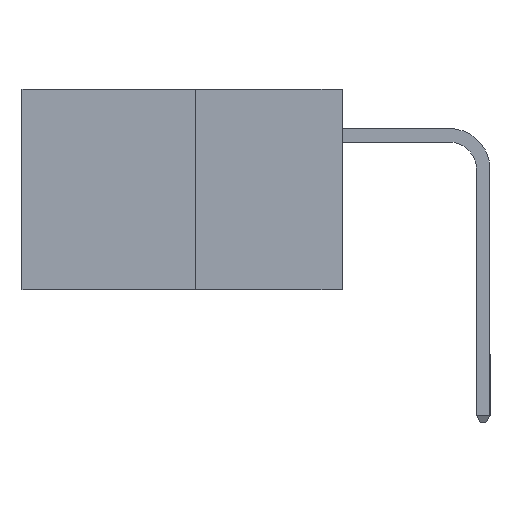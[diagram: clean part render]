
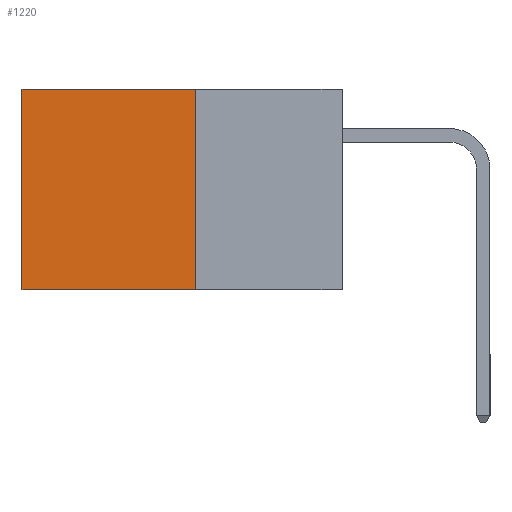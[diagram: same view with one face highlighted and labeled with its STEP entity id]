
A CAD part, left-side view. The second image highlights one B-rep face of the part: STEP entity #1220.
In plain terms, the highlighted planar face has unit normal (-1, 0, 0).
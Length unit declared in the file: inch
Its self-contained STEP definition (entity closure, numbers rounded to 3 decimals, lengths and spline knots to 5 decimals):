
#165 = LINE ( 'NONE', #10341, #7645 ) ;
#206 = CARTESIAN_POINT ( 'NONE',  ( 0.277, 0.27, -0.37 ) ) ;
#875 = EDGE_CURVE ( 'NONE', #8122, #924, #165, .T. ) ;
#924 = VERTEX_POINT ( 'NONE', #4427 ) ;
#1058 = ORIENTED_EDGE ( 'NONE', *, *, #8032, .T. ) ;
#1220 = ADVANCED_FACE ( 'NONE', ( #4016 ), #4090, .F. ) ;
#1400 = DIRECTION ( 'NONE',  ( 0., 0., -1. ) ) ;
#1431 = DIRECTION ( 'NONE',  ( 1., 0., 0. ) ) ;
#1976 = ORIENTED_EDGE ( 'NONE', *, *, #875, .F. ) ;
#2445 = LINE ( 'NONE', #11500, #9314 ) ;
#2619 = VECTOR ( 'NONE', #3828, 39.37008 ) ;
#2685 = AXIS2_PLACEMENT_3D ( 'NONE', #206, #1431, #1400 ) ;
#3040 = LINE ( 'NONE', #6504, #5522 ) ;
#3828 = DIRECTION ( 'NONE',  ( 0., 1., 0. ) ) ;
#4016 = FACE_OUTER_BOUND ( 'NONE', #5751, .T. ) ;
#4090 = PLANE ( 'NONE',  #2685 ) ;
#4427 = CARTESIAN_POINT ( 'NONE',  ( 0.277, 0.27, -0.37 ) ) ;
#4840 = CARTESIAN_POINT ( 'NONE',  ( 0.277, 0.27, 0. ) ) ;
#5522 = VECTOR ( 'NONE', #7401, 39.37008 ) ;
#5670 = ORIENTED_EDGE ( 'NONE', *, *, #6732, .T. ) ;
#5751 = EDGE_LOOP ( 'NONE', ( #1058, #10531, #1976, #5670 ) ) ;
#5807 = VERTEX_POINT ( 'NONE', #10992 ) ;
#6084 = VERTEX_POINT ( 'NONE', #8508 ) ;
#6504 = CARTESIAN_POINT ( 'NONE',  ( 0.277, 0.59, -0.37 ) ) ;
#6732 = EDGE_CURVE ( 'NONE', #8122, #5807, #7469, .T. ) ;
#6827 = EDGE_CURVE ( 'NONE', #924, #6084, #2445, .T. ) ;
#7401 = DIRECTION ( 'NONE',  ( 0., 0., -1. ) ) ;
#7469 = LINE ( 'NONE', #4840, #2619 ) ;
#7645 = VECTOR ( 'NONE', #10375, 39.37008 ) ;
#8032 = EDGE_CURVE ( 'NONE', #5807, #6084, #3040, .T. ) ;
#8122 = VERTEX_POINT ( 'NONE', #10058 ) ;
#8508 = CARTESIAN_POINT ( 'NONE',  ( 0.277, 0.59, -0.37 ) ) ;
#9314 = VECTOR ( 'NONE', #11193, 39.37008 ) ;
#10058 = CARTESIAN_POINT ( 'NONE',  ( 0.277, 0.27, 0. ) ) ;
#10341 = CARTESIAN_POINT ( 'NONE',  ( 0.277, 0.27, -0.37 ) ) ;
#10375 = DIRECTION ( 'NONE',  ( 0., 0., -1. ) ) ;
#10531 = ORIENTED_EDGE ( 'NONE', *, *, #6827, .F. ) ;
#10992 = CARTESIAN_POINT ( 'NONE',  ( 0.277, 0.59, 0. ) ) ;
#11193 = DIRECTION ( 'NONE',  ( 0., 1., 0. ) ) ;
#11500 = CARTESIAN_POINT ( 'NONE',  ( 0.277, 0.27, -0.37 ) ) ;
